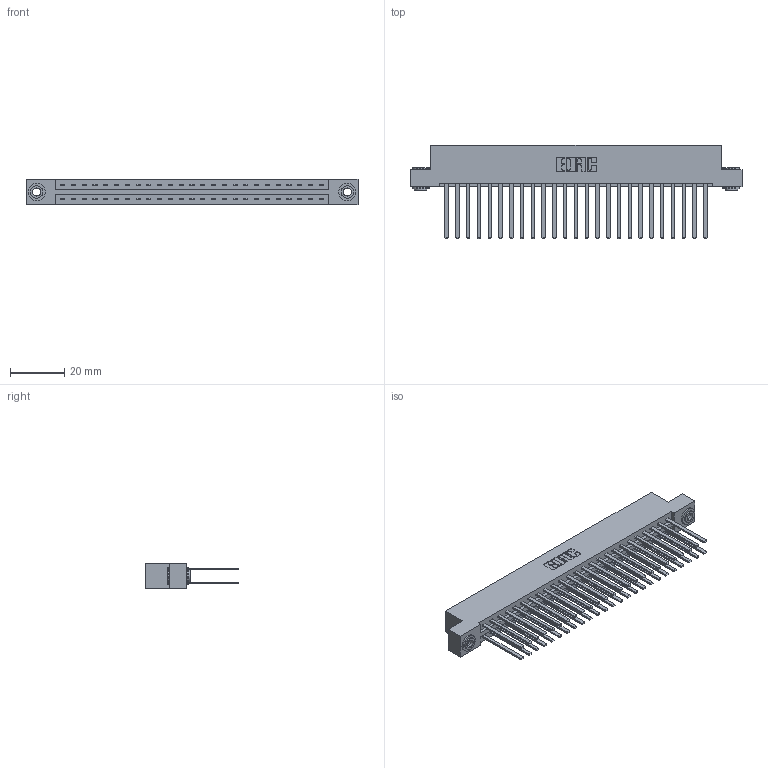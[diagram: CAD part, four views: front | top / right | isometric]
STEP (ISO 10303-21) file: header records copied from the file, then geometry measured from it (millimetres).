
FILE_DESCRIPTION (( 'STEP AP203' ), '1' );
FILE_NAME ('387-050-544-203.STEP', '2018-09-20T08:30:35', ( '' ), ( '' ), 'SwSTEP 2.0', 'SolidWorks 2016', '' );
FILE_SCHEMA (( 'CONFIG_CONTROL_DESIGN' ));
Length unit declared in the file: inch
Products named in the file (4): 337 Part_Flush Mounting Lugs - 0.156 Dia-TH; 345-292-001_345-293-144; 345-250-002_345-250-002-102; 387-050-544-203
Assembly tree (53 placements, depth 2):
  387-050-544-203
    337 Part_Flush Mounting Lugs - 0.156 Dia-TH
    345-292-001_345-293-144  x50
    345-250-002_345-250-002-102  x2
Bounding box: 122.07 x 34.3 x 9.4 mm (x, y, z)
Volume: 13359 mm3; surface area: 17451.3 mm2
Topology: 53 solids, 53 shells, 2552 faces, 7537 edges, 4954 vertices
Faces by surface type: plane 1780, cylinder 764, cone 8
Entity records: 22048 total; most frequent: CARTESIAN_POINT 3701, ORIENTED_EDGE 3630, DIRECTION 3209, EDGE_CURVE 1815, LINE 1667, VECTOR 1667, VERTEX_POINT 1206, AXIS2_PLACEMENT_3D 771
